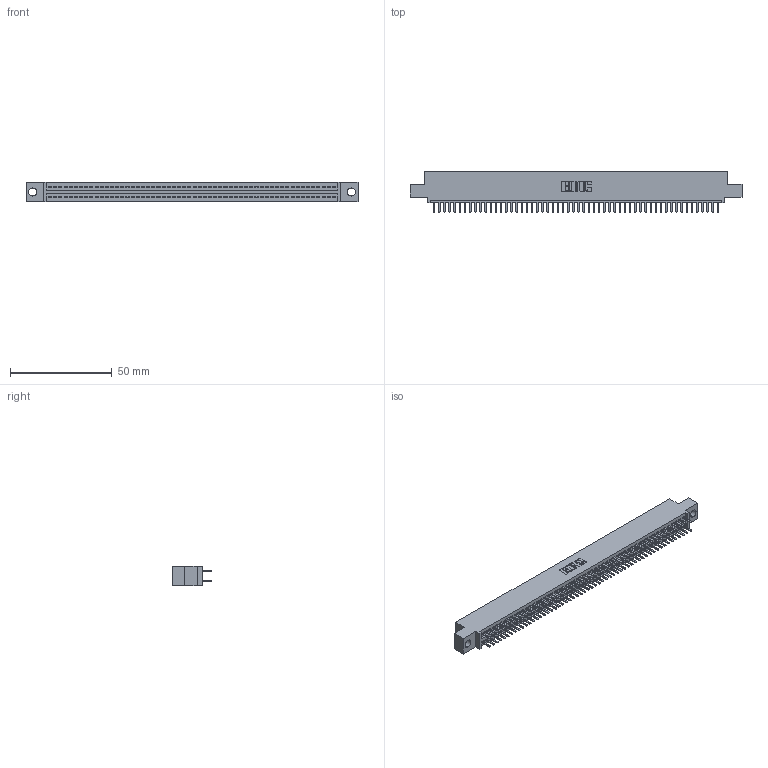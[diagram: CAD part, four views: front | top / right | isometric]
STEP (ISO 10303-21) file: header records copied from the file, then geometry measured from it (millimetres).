
FILE_DESCRIPTION (( 'STEP AP203' ), '1' );
FILE_NAME ('395-112-520-504.STEP', '2021-06-17T18:03:56', ( '' ), ( '' ), 'SwSTEP 2.0', 'SolidWorks 2020', '' );
FILE_SCHEMA (( 'CONFIG_CONTROL_DESIGN' ));
Length unit declared in the file: inch
Products named in the file (3): 345-292-001_345-293-120; 395-112-520-504; 345 Part_0.110 Offset - 0.156 Dia-TI
Assembly tree (113 placements, depth 2):
  395-112-520-504
    345 Part_0.110 Offset - 0.156 Dia-TI
    345-292-001_345-293-120  x112
Bounding box: 163.45 x 19.68 x 9.4 mm (x, y, z)
Volume: 15779 mm3; surface area: 23434.9 mm2
Topology: 113 solids, 113 shells, 6192 faces, 17973 edges, 11682 vertices
Faces by surface type: plane 4018, cylinder 2174
Entity records: 42719 total; most frequent: CARTESIAN_POINT 7166, ORIENTED_EDGE 7086, DIRECTION 6287, EDGE_CURVE 3543, VECTOR 3183, LINE 3183, VERTEX_POINT 2358, AXIS2_PLACEMENT_3D 1552
